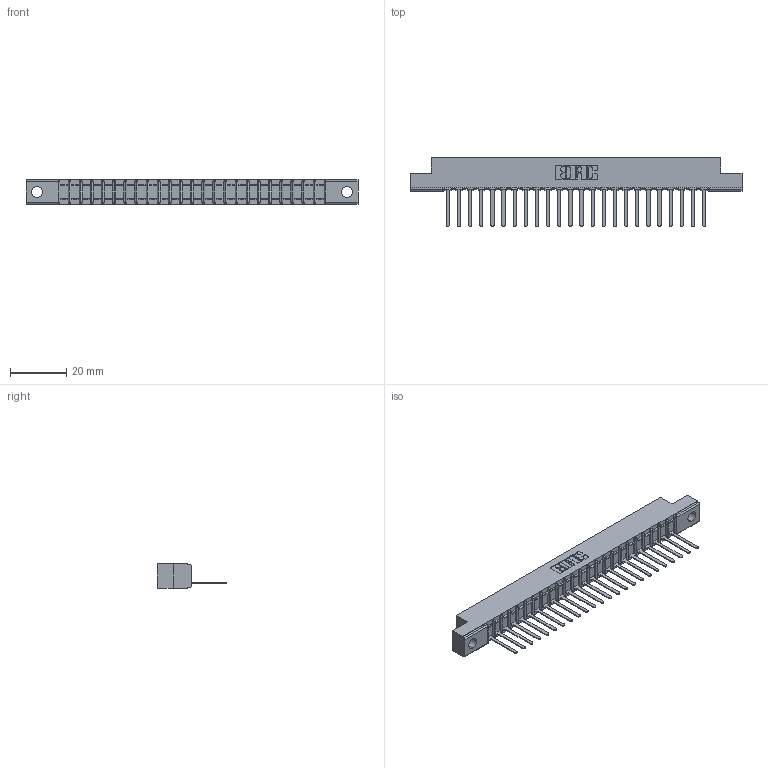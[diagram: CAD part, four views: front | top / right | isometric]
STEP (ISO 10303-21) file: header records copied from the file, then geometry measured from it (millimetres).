
FILE_DESCRIPTION (( 'STEP AP203' ), '1' );
FILE_NAME ('307-024-541-102.STEP', '2019-09-05T00:59:37', ( '' ), ( '' ), 'SwSTEP 2.0', 'SolidWorks 2016', '' );
FILE_SCHEMA (( 'CONFIG_CONTROL_DESIGN' ));
Length unit declared in the file: inch
Products named in the file (3): 307-024-541-102; 307-290-002_541; 307 Part_.128 Dia Mounting Holes
Assembly tree (25 placements, depth 2):
  307-024-541-102
    307 Part_.128 Dia Mounting Holes
    307-290-002_541  x24
Bounding box: 118.11 x 24.59 x 8.71 mm (x, y, z)
Volume: 7778.3 mm3; surface area: 14515.8 mm2
Topology: 25 solids, 25 shells, 1919 faces, 5891 edges, 3858 vertices
Faces by surface type: plane 1150, cylinder 719, sphere 50
Entity records: 23514 total; most frequent: CARTESIAN_POINT 3964, ORIENTED_EDGE 3954, DIRECTION 3859, EDGE_CURVE 1977, VECTOR 1505, LINE 1505, VERTEX_POINT 1282, AXIS2_PLACEMENT_3D 1177
